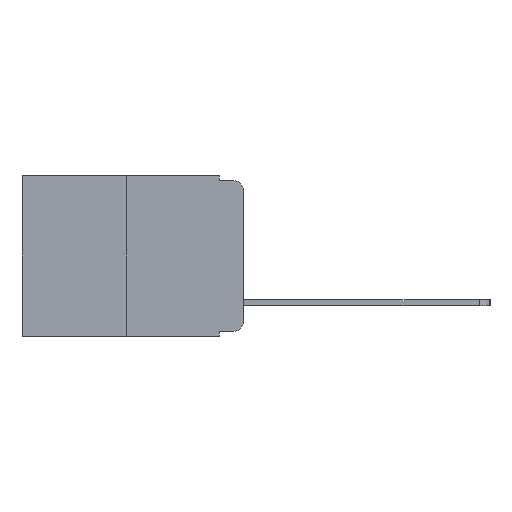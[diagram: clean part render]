
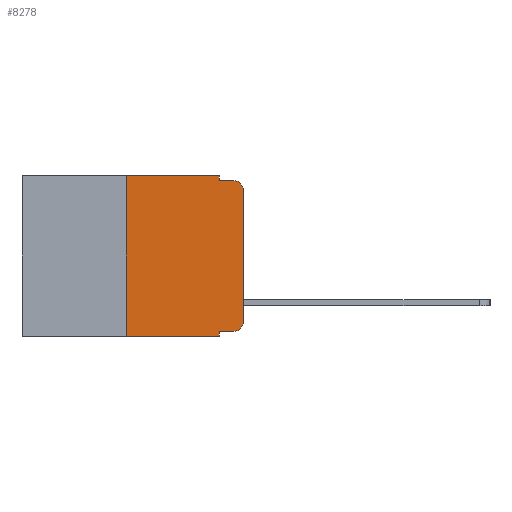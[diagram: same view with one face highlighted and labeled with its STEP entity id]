
A CAD part, left-side view. The second image highlights one B-rep face of the part: STEP entity #8278.
In plain terms, the highlighted planar face has unit normal (-1, 0, 0).
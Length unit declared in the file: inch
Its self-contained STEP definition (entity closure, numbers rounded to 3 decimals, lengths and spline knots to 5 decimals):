
#270 = CARTESIAN_POINT ( 'NONE',  ( 0., 0.051, -0.333 ) ) ;
#494 = VERTEX_POINT ( 'NONE', #13741 ) ;
#564 = ORIENTED_EDGE ( 'NONE', *, *, #15684, .T. ) ;
#780 = CARTESIAN_POINT ( 'NONE',  ( 0., 0.02, -0.01 ) ) ;
#842 = EDGE_CURVE ( 'NONE', #2280, #494, #15547, .T. ) ;
#903 = CIRCLE ( 'NONE', #16923, 0.02 ) ;
#929 = EDGE_LOOP ( 'NONE', ( #11062, #18086, #12337, #2880, #7195, #14319, #564, #6035, #16432, #10022 ) ) ;
#1067 = VERTEX_POINT ( 'NONE', #17667 ) ;
#1278 = DIRECTION ( 'NONE',  ( 0., -1., 0. ) ) ;
#1306 = DIRECTION ( 'NONE',  ( -1., 0., 0. ) ) ;
#1371 = CARTESIAN_POINT ( 'NONE',  ( 0., 0.02, -0.03 ) ) ;
#1681 = DIRECTION ( 'NONE',  ( 0., -1., 0. ) ) ;
#2153 = CARTESIAN_POINT ( 'NONE',  ( 0., 0.051, -0.343 ) ) ;
#2280 = VERTEX_POINT ( 'NONE', #10721 ) ;
#2876 = EDGE_CURVE ( 'NONE', #2280, #12205, #8265, .T. ) ;
#2880 = ORIENTED_EDGE ( 'NONE', *, *, #5931, .F. ) ;
#2903 = DIRECTION ( 'NONE',  ( 0., 0., -1. ) ) ;
#2943 = LINE ( 'NONE', #8250, #6511 ) ;
#3884 = EDGE_CURVE ( 'NONE', #5177, #10512, #13780, .T. ) ;
#4719 = VERTEX_POINT ( 'NONE', #780 ) ;
#5177 = VERTEX_POINT ( 'NONE', #13038 ) ;
#5653 = CIRCLE ( 'NONE', #14553, 0.02 ) ;
#5711 = CARTESIAN_POINT ( 'NONE',  ( 0., 0., -0.313 ) ) ;
#5931 = EDGE_CURVE ( 'NONE', #5951, #1067, #18103, .T. ) ;
#5951 = VERTEX_POINT ( 'NONE', #17797 ) ;
#6035 = ORIENTED_EDGE ( 'NONE', *, *, #2876, .F. ) ;
#6132 = VECTOR ( 'NONE', #7523, 39.37008 ) ;
#6197 = VERTEX_POINT ( 'NONE', #18526 ) ;
#6511 = VECTOR ( 'NONE', #17902, 39.37008 ) ;
#6887 = CARTESIAN_POINT ( 'NONE',  ( 0., 0.473, 0. ) ) ;
#6953 = EDGE_CURVE ( 'NONE', #1067, #4719, #18404, .T. ) ;
#7195 = ORIENTED_EDGE ( 'NONE', *, *, #13446, .F. ) ;
#7357 = VECTOR ( 'NONE', #1278, 39.37008 ) ;
#7523 = DIRECTION ( 'NONE',  ( 0., 0., 1. ) ) ;
#7944 = EDGE_CURVE ( 'NONE', #6197, #4719, #5653, .T. ) ;
#8250 = CARTESIAN_POINT ( 'NONE',  ( 0., 0.473, 0. ) ) ;
#8265 = LINE ( 'NONE', #12234, #11686 ) ;
#8278 = ADVANCED_FACE ( 'NONE', ( #13764 ), #15339, .F. ) ;
#8355 = DIRECTION ( 'NONE',  ( 1., 0., 0. ) ) ;
#10022 = ORIENTED_EDGE ( 'NONE', *, *, #18449, .T. ) ;
#10332 = CARTESIAN_POINT ( 'NONE',  ( 0., 0.02, -0.313 ) ) ;
#10512 = VERTEX_POINT ( 'NONE', #10592 ) ;
#10592 = CARTESIAN_POINT ( 'NONE',  ( 0., 0.25, 0. ) ) ;
#10721 = CARTESIAN_POINT ( 'NONE',  ( 0., 0.051, -0.333 ) ) ;
#10899 = EDGE_CURVE ( 'NONE', #12870, #6197, #16550, .T. ) ;
#10962 = DIRECTION ( 'NONE',  ( 0., 0., -1. ) ) ;
#11062 = ORIENTED_EDGE ( 'NONE', *, *, #10899, .T. ) ;
#11349 = LINE ( 'NONE', #16215, #17657 ) ;
#11521 = VECTOR ( 'NONE', #1681, 39.37008 ) ;
#11686 = VECTOR ( 'NONE', #12531, 39.37008 ) ;
#11748 = DIRECTION ( 'NONE',  ( 0., 0., -1. ) ) ;
#11798 = DIRECTION ( 'NONE',  ( -1., 0., 0. ) ) ;
#12024 = CARTESIAN_POINT ( 'NONE',  ( 0., 0.25, 0. ) ) ;
#12205 = VERTEX_POINT ( 'NONE', #2153 ) ;
#12234 = CARTESIAN_POINT ( 'NONE',  ( 0., 0.051, 0. ) ) ;
#12337 = ORIENTED_EDGE ( 'NONE', *, *, #6953, .F. ) ;
#12531 = DIRECTION ( 'NONE',  ( 0., 0., -1. ) ) ;
#12870 = VERTEX_POINT ( 'NONE', #5711 ) ;
#12926 = CARTESIAN_POINT ( 'NONE',  ( 0., 0., 0. ) ) ;
#13038 = CARTESIAN_POINT ( 'NONE',  ( 0., 0.25, -0.343 ) ) ;
#13446 = EDGE_CURVE ( 'NONE', #10512, #5951, #2943, .T. ) ;
#13741 = CARTESIAN_POINT ( 'NONE',  ( 0., 0.02, -0.333 ) ) ;
#13764 = FACE_OUTER_BOUND ( 'NONE', #929, .T. ) ;
#13780 = LINE ( 'NONE', #12024, #6132 ) ;
#13828 = VECTOR ( 'NONE', #14283, 39.37008 ) ;
#13885 = AXIS2_PLACEMENT_3D ( 'NONE', #6887, #8355, #18016 ) ;
#13999 = DIRECTION ( 'NONE',  ( 0., -1., 0. ) ) ;
#14283 = DIRECTION ( 'NONE',  ( 0., 0., 1. ) ) ;
#14319 = ORIENTED_EDGE ( 'NONE', *, *, #3884, .F. ) ;
#14553 = AXIS2_PLACEMENT_3D ( 'NONE', #1371, #11798, #2903 ) ;
#14556 = VECTOR ( 'NONE', #10962, 39.37008 ) ;
#15339 = PLANE ( 'NONE',  #13885 ) ;
#15547 = LINE ( 'NONE', #270, #11521 ) ;
#15684 = EDGE_CURVE ( 'NONE', #5177, #12205, #11349, .T. ) ;
#16215 = CARTESIAN_POINT ( 'NONE',  ( 0., 0.473, -0.343 ) ) ;
#16356 = CARTESIAN_POINT ( 'NONE',  ( 0., 0.051, 0. ) ) ;
#16432 = ORIENTED_EDGE ( 'NONE', *, *, #842, .T. ) ;
#16550 = LINE ( 'NONE', #12926, #13828 ) ;
#16923 = AXIS2_PLACEMENT_3D ( 'NONE', #10332, #1306, #11748 ) ;
#17657 = VECTOR ( 'NONE', #13999, 39.37008 ) ;
#17667 = CARTESIAN_POINT ( 'NONE',  ( 0., 0.051, -0.01 ) ) ;
#17797 = CARTESIAN_POINT ( 'NONE',  ( 0., 0.051, 0. ) ) ;
#17902 = DIRECTION ( 'NONE',  ( 0., -1., 0. ) ) ;
#18016 = DIRECTION ( 'NONE',  ( 0., 0., -1. ) ) ;
#18086 = ORIENTED_EDGE ( 'NONE', *, *, #7944, .T. ) ;
#18103 = LINE ( 'NONE', #16356, #14556 ) ;
#18336 = CARTESIAN_POINT ( 'NONE',  ( 0., 0.051, -0.01 ) ) ;
#18404 = LINE ( 'NONE', #18336, #7357 ) ;
#18449 = EDGE_CURVE ( 'NONE', #494, #12870, #903, .T. ) ;
#18526 = CARTESIAN_POINT ( 'NONE',  ( 0., 0., -0.03 ) ) ;
